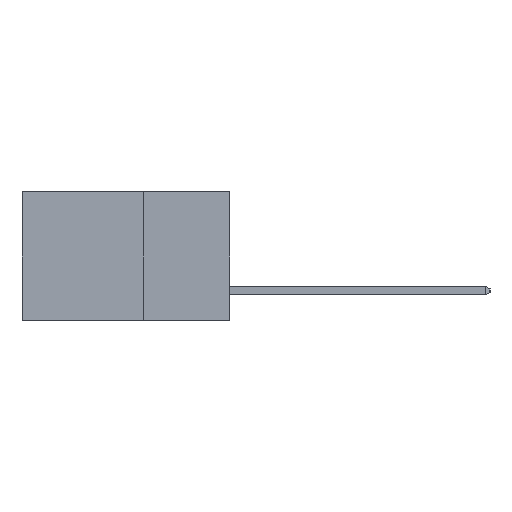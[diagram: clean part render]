
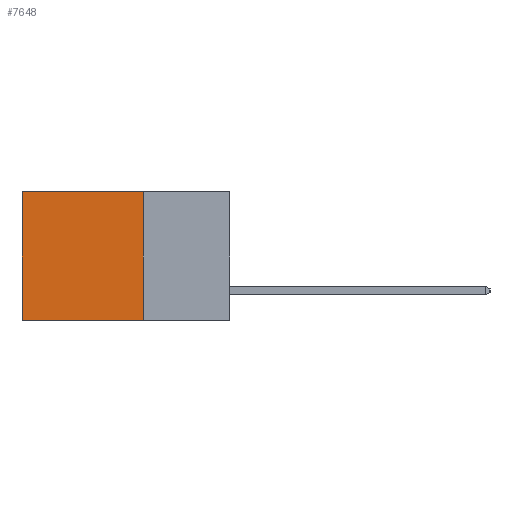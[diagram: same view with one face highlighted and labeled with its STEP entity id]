
A CAD part, left-side view. The second image highlights one B-rep face of the part: STEP entity #7648.
In plain terms, the highlighted planar face has unit normal (-1, 0, 0).
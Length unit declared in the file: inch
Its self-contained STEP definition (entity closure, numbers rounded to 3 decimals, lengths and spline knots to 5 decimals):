
#92 = EDGE_CURVE ( 'NONE', #10829, #6186, #163, .T. ) ;
#163 = LINE ( 'NONE', #6524, #4868 ) ;
#212 = EDGE_CURVE ( 'NONE', #7670, #6186, #5827, .T. ) ;
#232 = DIRECTION ( 'NONE',  ( 0., 0., -1. ) ) ;
#344 = CARTESIAN_POINT ( 'NONE',  ( 0.2615, 0.6, -0.37 ) ) ;
#468 = DIRECTION ( 'NONE',  ( 1., 0., 0. ) ) ;
#997 = EDGE_CURVE ( 'NONE', #1764, #10829, #1059, .T. ) ;
#1059 = LINE ( 'NONE', #2555, #9759 ) ;
#1156 = ORIENTED_EDGE ( 'NONE', *, *, #997, .F. ) ;
#1211 = LINE ( 'NONE', #2164, #5806 ) ;
#1448 = CARTESIAN_POINT ( 'NONE',  ( 0.2615, 0.6, 0. ) ) ;
#1764 = VERTEX_POINT ( 'NONE', #10242 ) ;
#1771 = ORIENTED_EDGE ( 'NONE', *, *, #92, .F. ) ;
#2164 = CARTESIAN_POINT ( 'NONE',  ( 0.2615, 0.25, 0. ) ) ;
#2210 = FACE_OUTER_BOUND ( 'NONE', #2314, .T. ) ;
#2314 = EDGE_LOOP ( 'NONE', ( #2687, #1771, #1156, #7736 ) ) ;
#2555 = CARTESIAN_POINT ( 'NONE',  ( 0.2615, 0.25, -0.37 ) ) ;
#2687 = ORIENTED_EDGE ( 'NONE', *, *, #212, .T. ) ;
#3041 = DIRECTION ( 'NONE',  ( 0., 0., -1. ) ) ;
#3194 = CARTESIAN_POINT ( 'NONE',  ( 0.2615, 0.25, -0.37 ) ) ;
#3582 = VECTOR ( 'NONE', #232, 39.37008 ) ;
#3914 = DIRECTION ( 'NONE',  ( 0., 1., 0. ) ) ;
#4868 = VECTOR ( 'NONE', #3914, 39.37008 ) ;
#5466 = CARTESIAN_POINT ( 'NONE',  ( 0.2615, 0.25, -0.37 ) ) ;
#5546 = DIRECTION ( 'NONE',  ( 0., 1., 0. ) ) ;
#5743 = PLANE ( 'NONE',  #6249 ) ;
#5806 = VECTOR ( 'NONE', #5546, 39.37008 ) ;
#5827 = LINE ( 'NONE', #6697, #3582 ) ;
#6186 = VERTEX_POINT ( 'NONE', #344 ) ;
#6249 = AXIS2_PLACEMENT_3D ( 'NONE', #3194, #468, #6571 ) ;
#6524 = CARTESIAN_POINT ( 'NONE',  ( 0.2615, 0.25, -0.37 ) ) ;
#6571 = DIRECTION ( 'NONE',  ( 0., 0., -1. ) ) ;
#6697 = CARTESIAN_POINT ( 'NONE',  ( 0.2615, 0.6, -0.37 ) ) ;
#7509 = EDGE_CURVE ( 'NONE', #1764, #7670, #1211, .T. ) ;
#7648 = ADVANCED_FACE ( 'NONE', ( #2210 ), #5743, .F. ) ;
#7670 = VERTEX_POINT ( 'NONE', #1448 ) ;
#7736 = ORIENTED_EDGE ( 'NONE', *, *, #7509, .T. ) ;
#9759 = VECTOR ( 'NONE', #3041, 39.37008 ) ;
#10242 = CARTESIAN_POINT ( 'NONE',  ( 0.2615, 0.25, 0. ) ) ;
#10829 = VERTEX_POINT ( 'NONE', #5466 ) ;
